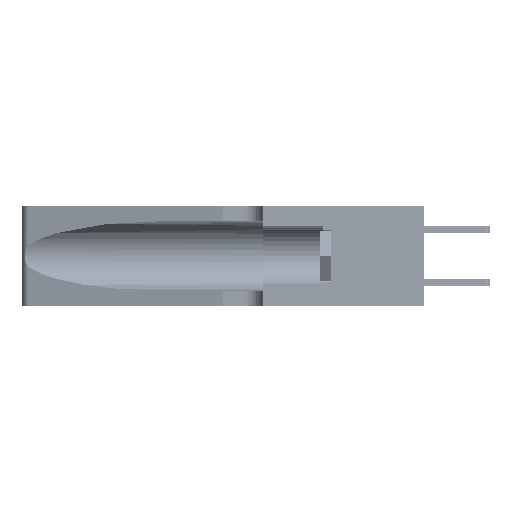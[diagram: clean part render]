
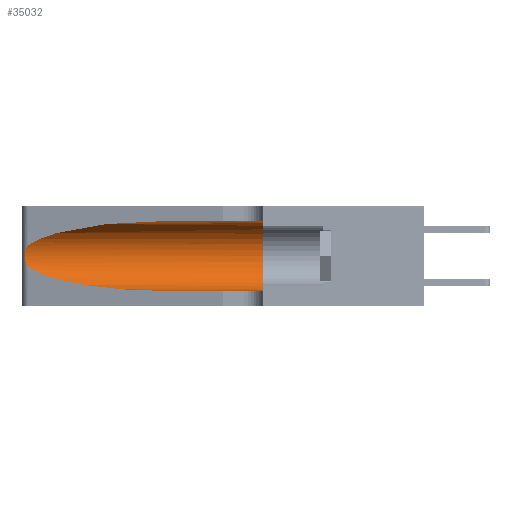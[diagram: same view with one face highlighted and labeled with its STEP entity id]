
A CAD part, left-side view. The second image highlights one B-rep face of the part: STEP entity #35032.
In plain terms, the highlighted cylindrical face has radius 3.308 mm (diameter 6.617 mm), a partial arc.
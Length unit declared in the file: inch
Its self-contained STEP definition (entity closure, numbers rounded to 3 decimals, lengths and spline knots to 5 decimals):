
#828 = EDGE_CURVE ( 'NONE', #32914, #43219, #6592, .T. ) ;
#1438 = EDGE_LOOP ( 'NONE', ( #19413, #7991, #10349, #14410, #2751, #28319 ) ) ;
#1644 = CARTESIAN_POINT ( 'NONE',  ( 0.25555, 1.22994, 0.2215 ) ) ;
#2751 = ORIENTED_EDGE ( 'NONE', *, *, #41338, .F. ) ;
#2925 = CARTESIAN_POINT ( 'NONE',  ( 0.1305, 0.72297, 0.31525 ) ) ;
#3639 = CARTESIAN_POINT ( 'NONE',  ( 0.1305, 0.72297, 0.31525 ) ) ;
#4511 = EDGE_CURVE ( 'NONE', #12920, #32914, #45608, .T. ) ;
#4542 = CARTESIAN_POINT ( 'NONE',  ( 0.25487, 1.22718, 0.14631 ) ) ;
#4770 = VECTOR ( 'NONE', #13594, 39.37008 ) ;
#6592 =( BOUNDED_CURVE ( )  B_SPLINE_CURVE ( 3, ( #4542, #37495, #33960, #15144 ),
 .UNSPECIFIED., .F., .F. ) 
 B_SPLINE_CURVE_WITH_KNOTS ( ( 4, 4 ),
 ( 3.44316, 4.71239 ),
 .UNSPECIFIED. ) 
 CURVE ( )  GEOMETRIC_REPRESENTATION_ITEM ( )  RATIONAL_B_SPLINE_CURVE ( ( 1., 0.87, 0.87, 1. ) ) 
 REPRESENTATION_ITEM ( '' )  );
#7991 = ORIENTED_EDGE ( 'NONE', *, *, #4511, .T. ) ;
#9939 = CARTESIAN_POINT ( 'NONE',  ( 0.25487, 1.22718, 0.14631 ) ) ;
#9974 = AXIS2_PLACEMENT_3D ( 'NONE', #22734, #34079, #34237 ) ;
#10267 = CARTESIAN_POINT ( 'NONE',  ( 0.25487, 1.22718, 0.22369 ) ) ;
#10349 = ORIENTED_EDGE ( 'NONE', *, *, #828, .T. ) ;
#12326 = DIRECTION ( 'NONE',  ( 0., 0., -1. ) ) ;
#12920 = VERTEX_POINT ( 'NONE', #38282 ) ;
#12958 = CARTESIAN_POINT ( 'NONE',  ( 0.1305, 1.61858, 0.185 ) ) ;
#13594 = DIRECTION ( 'NONE',  ( 0., -1., 0. ) ) ;
#13640 = CARTESIAN_POINT ( 'NONE',  ( 0.25555, 1.22993, 0.14849 ) ) ;
#13800 = CARTESIAN_POINT ( 'NONE',  ( 0.26017, 1.23833, 0.17102 ) ) ;
#14296 = CARTESIAN_POINT ( 'NONE',  ( 0.1305, 0.35, 0.31525 ) ) ;
#14410 = ORIENTED_EDGE ( 'NONE', *, *, #46736, .T. ) ;
#14638 = VERTEX_POINT ( 'NONE', #40010 ) ;
#15144 = CARTESIAN_POINT ( 'NONE',  ( 0.1305, 0.72297, 0.05475 ) ) ;
#17156 = CARTESIAN_POINT ( 'NONE',  ( 0.25639, 1.23186, 0.15144 ) ) ;
#17317 = CARTESIAN_POINT ( 'NONE',  ( 0.26075, 1.23896, 0.19203 ) ) ;
#17461 = CARTESIAN_POINT ( 'NONE',  ( 0.26018, 1.23835, 0.19895 ) ) ;
#19413 = ORIENTED_EDGE ( 'NONE', *, *, #44419, .T. ) ;
#19417 = FACE_OUTER_BOUND ( 'NONE', #1438, .T. ) ;
#19994 = DIRECTION ( 'NONE',  ( 0., -1., 0. ) ) ;
#21314 = CARTESIAN_POINT ( 'NONE',  ( 0.25787, 1.23484, 0.2124 ) ) ;
#22734 = CARTESIAN_POINT ( 'NONE',  ( 0.1305, 0.35, 0.185 ) ) ;
#24019 = CYLINDRICAL_SURFACE ( 'NONE', #32154, 0.13025 ) ;
#24969 = VERTEX_POINT ( 'NONE', #3639 ) ;
#28319 = ORIENTED_EDGE ( 'NONE', *, *, #37855, .F. ) ;
#28321 = CARTESIAN_POINT ( 'NONE',  ( 0.25789, 1.23486, 0.15765 ) ) ;
#31226 = LINE ( 'NONE', #46810, #40951 ) ;
#31840 = CARTESIAN_POINT ( 'NONE',  ( 0.25854, 1.2359, 0.20912 ) ) ;
#32154 = AXIS2_PLACEMENT_3D ( 'NONE', #12958, #19994, #12326 ) ;
#32488 = CARTESIAN_POINT ( 'NONE',  ( 0.2373, 1.15595, 0.28018 ) ) ;
#32644 = CARTESIAN_POINT ( 'NONE',  ( 0.18966, 0.96281, 0.31525 ) ) ;
#32914 = VERTEX_POINT ( 'NONE', #34210 ) ;
#33960 = CARTESIAN_POINT ( 'NONE',  ( 0.18966, 0.96281, 0.05475 ) ) ;
#34079 = DIRECTION ( 'NONE',  ( 0., 1., 0. ) ) ;
#34210 = CARTESIAN_POINT ( 'NONE',  ( 0.25487, 1.22718, 0.14631 ) ) ;
#34237 = DIRECTION ( 'NONE',  ( 0., 0., 1. ) ) ;
#35032 = ADVANCED_FACE ( 'NONE', ( #19417 ), #24019, .F. ) ;
#35543 = CARTESIAN_POINT ( 'NONE',  ( 0.25856, 1.23593, 0.16098 ) ) ;
#35929 = DIRECTION ( 'NONE',  ( 0., -1., 0. ) ) ;
#37495 = CARTESIAN_POINT ( 'NONE',  ( 0.2373, 1.15595, 0.08982 ) ) ;
#37855 = EDGE_CURVE ( 'NONE', #24969, #42347, #31226, .T. ) ;
#38282 = CARTESIAN_POINT ( 'NONE',  ( 0.25487, 1.22718, 0.22369 ) ) ;
#39170 = CARTESIAN_POINT ( 'NONE',  ( 0.1305, 1.61858, 0.05475 ) ) ;
#39968 = CARTESIAN_POINT ( 'NONE',  ( 0.1305, 0.72297, 0.05475 ) ) ;
#40010 = CARTESIAN_POINT ( 'NONE',  ( 0.1305, 0.35, 0.05475 ) ) ;
#40951 = VECTOR ( 'NONE', #35929, 39.37008 ) ;
#41328 = CIRCLE ( 'NONE', #9974, 0.13025 ) ;
#41338 = EDGE_CURVE ( 'NONE', #42347, #14638, #41328, .T. ) ;
#42256 = CARTESIAN_POINT ( 'NONE',  ( 0.25487, 1.22718, 0.22369 ) ) ;
#42347 = VERTEX_POINT ( 'NONE', #14296 ) ;
#42729 =( BOUNDED_CURVE ( )  B_SPLINE_CURVE ( 3, ( #2925, #32644, #32488, #10267 ),
 .UNSPECIFIED., .F., .T. ) 
 B_SPLINE_CURVE_WITH_KNOTS ( ( 4, 4 ),
 ( 1.5708, 2.84003 ),
 .UNSPECIFIED. ) 
 CURVE ( )  GEOMETRIC_REPRESENTATION_ITEM ( )  RATIONAL_B_SPLINE_CURVE ( ( 1., 0.87, 0.87, 1. ) ) 
 REPRESENTATION_ITEM ( '' )  );
#43077 = CARTESIAN_POINT ( 'NONE',  ( 0.26075, 1.23896, 0.178 ) ) ;
#43219 = VERTEX_POINT ( 'NONE', #39968 ) ;
#44419 = EDGE_CURVE ( 'NONE', #24969, #12920, #42729, .T. ) ;
#45608 = B_SPLINE_CURVE_WITH_KNOTS ( 'NONE', 3,
 ( #42256, #1644, #46284, #21314, #31840, #17461, #17317, #43077, #13800, #35543, #28321, #17156, #13640, #9939 ),
 .UNSPECIFIED., .F., .F.,
 ( 4, 2, 2, 2, 2, 2, 4 ),
 ( 0., 0.00027, 0.00053, 0.00107, 0.0016, 0.00187, 0.00214 ),
 .UNSPECIFIED. ) ;
#46284 = CARTESIAN_POINT ( 'NONE',  ( 0.25639, 1.23184, 0.21858 ) ) ;
#46555 = LINE ( 'NONE', #39170, #4770 ) ;
#46736 = EDGE_CURVE ( 'NONE', #43219, #14638, #46555, .T. ) ;
#46810 = CARTESIAN_POINT ( 'NONE',  ( 0.1305, 1.61858, 0.31525 ) ) ;
